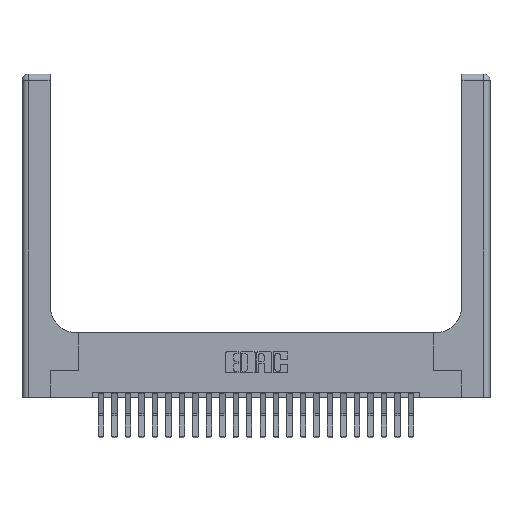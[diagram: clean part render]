
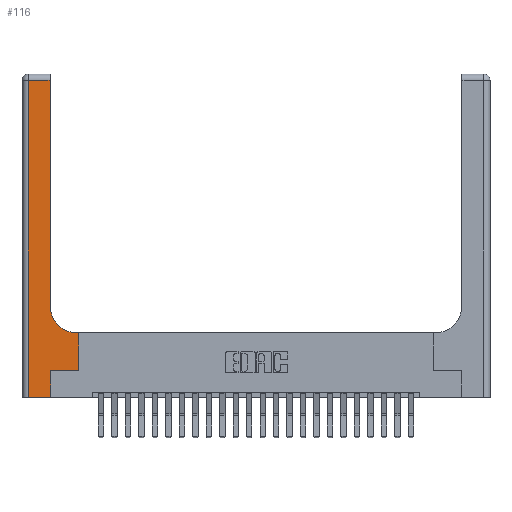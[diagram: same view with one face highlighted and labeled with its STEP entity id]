
A CAD part, top view. The second image highlights one B-rep face of the part: STEP entity #116.
In plain terms, the highlighted planar face has unit normal (0, 0, 1).
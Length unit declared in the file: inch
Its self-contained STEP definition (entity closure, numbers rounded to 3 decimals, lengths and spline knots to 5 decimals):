
#116 = ADVANCED_FACE ( 'NONE', ( #17686 ), #1300, .F. ) ;
#833 = LINE ( 'NONE', #8293, #1927 ) ;
#1001 = VERTEX_POINT ( 'NONE', #23063 ) ;
#1300 = PLANE ( 'NONE',  #13928 ) ;
#1876 = DIRECTION ( 'NONE',  ( 1., 0., 0. ) ) ;
#1925 = AXIS2_PLACEMENT_3D ( 'NONE', #21440, #13612, #12047 ) ;
#1927 = VECTOR ( 'NONE', #7941, 39.37008 ) ;
#2164 = EDGE_CURVE ( 'NONE', #12956, #5318, #8235, .T. ) ;
#2205 = ORIENTED_EDGE ( 'NONE', *, *, #17140, .T. ) ;
#2986 = VECTOR ( 'NONE', #16408, 39.37008 ) ;
#3011 = EDGE_CURVE ( 'NONE', #8591, #12956, #19226, .T. ) ;
#5019 = ORIENTED_EDGE ( 'NONE', *, *, #10632, .T. ) ;
#5085 = VERTEX_POINT ( 'NONE', #17331 ) ;
#5103 = ORIENTED_EDGE ( 'NONE', *, *, #19795, .T. ) ;
#5318 = VERTEX_POINT ( 'NONE', #16356 ) ;
#5699 = VERTEX_POINT ( 'NONE', #7282 ) ;
#6354 = VERTEX_POINT ( 'NONE', #15540 ) ;
#7282 = CARTESIAN_POINT ( 'NONE',  ( 0.528, 0.6, 0.37 ) ) ;
#7941 = DIRECTION ( 'NONE',  ( 0., 1., 0. ) ) ;
#7951 = LINE ( 'NONE', #11822, #22887 ) ;
#8235 = LINE ( 'NONE', #12443, #14165 ) ;
#8293 = CARTESIAN_POINT ( 'NONE',  ( 0.265, 0., 0.37 ) ) ;
#8551 = LINE ( 'NONE', #19882, #15055 ) ;
#8591 = VERTEX_POINT ( 'NONE', #19841 ) ;
#8755 = DIRECTION ( 'NONE',  ( 0., 0., -1. ) ) ;
#8924 = CARTESIAN_POINT ( 'NONE',  ( 0.26, 0.6, 0.37 ) ) ;
#9002 = EDGE_CURVE ( 'NONE', #5085, #6354, #7951, .T. ) ;
#9160 = VECTOR ( 'NONE', #22289, 39.37008 ) ;
#9220 = LINE ( 'NONE', #20079, #10653 ) ;
#9275 = CARTESIAN_POINT ( 'NONE',  ( 0., 2.94, 0.37 ) ) ;
#10118 = VERTEX_POINT ( 'NONE', #16432 ) ;
#10632 = EDGE_CURVE ( 'NONE', #5699, #8591, #16167, .T. ) ;
#10653 = VECTOR ( 'NONE', #1876, 39.37008 ) ;
#10851 = DIRECTION ( 'NONE',  ( -1., 0., 0. ) ) ;
#11084 = LINE ( 'NONE', #20368, #9160 ) ;
#11822 = CARTESIAN_POINT ( 'NONE',  ( 0., 0., 0.37 ) ) ;
#11869 = EDGE_CURVE ( 'NONE', #5318, #10118, #16396, .T. ) ;
#12047 = DIRECTION ( 'NONE',  ( 1., 0., 0. ) ) ;
#12443 = CARTESIAN_POINT ( 'NONE',  ( 0.26, 3., 0.37 ) ) ;
#12835 = EDGE_CURVE ( 'NONE', #21711, #1001, #9220, .T. ) ;
#12956 = VERTEX_POINT ( 'NONE', #15365 ) ;
#13498 = DIRECTION ( 'NONE',  ( 1., 0., 0. ) ) ;
#13612 = DIRECTION ( 'NONE',  ( 0., 0., -1. ) ) ;
#13928 = AXIS2_PLACEMENT_3D ( 'NONE', #15884, #8755, #16119 ) ;
#14011 = VECTOR ( 'NONE', #10851, 39.37008 ) ;
#14165 = VECTOR ( 'NONE', #23412, 39.37008 ) ;
#14336 = DIRECTION ( 'NONE',  ( 0., -1., 0. ) ) ;
#14640 = ORIENTED_EDGE ( 'NONE', *, *, #3011, .T. ) ;
#15055 = VECTOR ( 'NONE', #14336, 39.37008 ) ;
#15365 = CARTESIAN_POINT ( 'NONE',  ( 0.26, 0.85, 0.37 ) ) ;
#15540 = CARTESIAN_POINT ( 'NONE',  ( 0.265, 0., 0.37 ) ) ;
#15884 = CARTESIAN_POINT ( 'NONE',  ( 0., 3., 0.37 ) ) ;
#16119 = DIRECTION ( 'NONE',  ( -1., 0., 0. ) ) ;
#16167 = LINE ( 'NONE', #8924, #2986 ) ;
#16335 = ORIENTED_EDGE ( 'NONE', *, *, #17247, .T. ) ;
#16356 = CARTESIAN_POINT ( 'NONE',  ( 0.26, 2.94, 0.37 ) ) ;
#16396 = LINE ( 'NONE', #9275, #14011 ) ;
#16408 = DIRECTION ( 'NONE',  ( -1., 0., 0. ) ) ;
#16432 = CARTESIAN_POINT ( 'NONE',  ( 0.06, 2.94, 0.37 ) ) ;
#16695 = ORIENTED_EDGE ( 'NONE', *, *, #9002, .T. ) ;
#17140 = EDGE_CURVE ( 'NONE', #10118, #5085, #8551, .T. ) ;
#17247 = EDGE_CURVE ( 'NONE', #1001, #5699, #11084, .T. ) ;
#17331 = CARTESIAN_POINT ( 'NONE',  ( 0.06, 0., 0.37 ) ) ;
#17686 = FACE_OUTER_BOUND ( 'NONE', #21159, .T. ) ;
#19101 = ORIENTED_EDGE ( 'NONE', *, *, #12835, .T. ) ;
#19226 = CIRCLE ( 'NONE', #1925, 0.25 ) ;
#19708 = ORIENTED_EDGE ( 'NONE', *, *, #2164, .T. ) ;
#19795 = EDGE_CURVE ( 'NONE', #6354, #21711, #833, .T. ) ;
#19841 = CARTESIAN_POINT ( 'NONE',  ( 0.51, 0.6, 0.37 ) ) ;
#19882 = CARTESIAN_POINT ( 'NONE',  ( 0.06, 3., 0.37 ) ) ;
#20079 = CARTESIAN_POINT ( 'NONE',  ( 0.265, 0.25, 0.37 ) ) ;
#20368 = CARTESIAN_POINT ( 'NONE',  ( 0.528, 0.25, 0.37 ) ) ;
#20562 = CARTESIAN_POINT ( 'NONE',  ( 0.265, 0.25, 0.37 ) ) ;
#21039 = ORIENTED_EDGE ( 'NONE', *, *, #11869, .T. ) ;
#21159 = EDGE_LOOP ( 'NONE', ( #19708, #21039, #2205, #16695, #5103, #19101, #16335, #5019, #14640 ) ) ;
#21440 = CARTESIAN_POINT ( 'NONE',  ( 0.51, 0.85, 0.37 ) ) ;
#21711 = VERTEX_POINT ( 'NONE', #20562 ) ;
#22289 = DIRECTION ( 'NONE',  ( 0., 1., 0. ) ) ;
#22887 = VECTOR ( 'NONE', #13498, 39.37008 ) ;
#23063 = CARTESIAN_POINT ( 'NONE',  ( 0.528, 0.25, 0.37 ) ) ;
#23412 = DIRECTION ( 'NONE',  ( 0., 1., 0. ) ) ;
